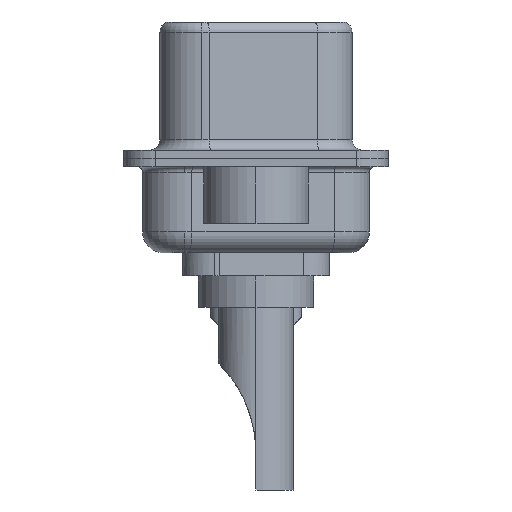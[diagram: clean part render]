
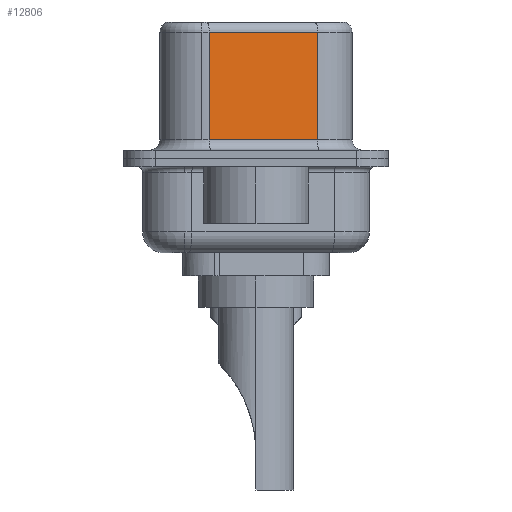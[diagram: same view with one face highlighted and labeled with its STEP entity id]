
A CAD part, left-side view. The second image highlights one B-rep face of the part: STEP entity #12806.
In plain terms, the highlighted planar face has unit normal (-0.985, -0.174, 0).
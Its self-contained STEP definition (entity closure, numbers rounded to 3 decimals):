
#2172 = CARTESIAN_POINT ( 'NONE',  ( 4.585, -2.927, 0.9 ) ) ;
#2495 = ORIENTED_EDGE ( 'NONE', *, *, #9477, .F. ) ;
#3134 = CARTESIAN_POINT ( 'NONE',  ( 3.675, 2.233, 6.02 ) ) ;
#3304 = VERTEX_POINT ( 'NONE', #3134 ) ;
#4158 = CARTESIAN_POINT ( 'NONE',  ( 4.585, -2.927, 0.9 ) ) ;
#4220 = VECTOR ( 'NONE', #18184, 1000. ) ;
#4547 = LINE ( 'NONE', #4779, #8338 ) ;
#4556 = EDGE_CURVE ( 'NONE', #10216, #3304, #4547, .T. ) ;
#4779 = CARTESIAN_POINT ( 'NONE',  ( 4.585, -2.927, 6.02 ) ) ;
#4795 = DIRECTION ( 'NONE',  ( 0.985, 0.174, 0. ) ) ;
#5337 = CARTESIAN_POINT ( 'NONE',  ( 4.585, -2.927, 6.52 ) ) ;
#7365 = DIRECTION ( 'NONE',  ( 0.174, -0.985, 0. ) ) ;
#8338 = VECTOR ( 'NONE', #15722, 1000. ) ;
#8511 = LINE ( 'NONE', #12081, #4220 ) ;
#9477 = EDGE_CURVE ( 'NONE', #10216, #18686, #19668, .T. ) ;
#10051 = ORIENTED_EDGE ( 'NONE', *, *, #4556, .T. ) ;
#10216 = VERTEX_POINT ( 'NONE', #19358 ) ;
#10341 = EDGE_CURVE ( 'NONE', #20203, #18686, #15147, .T. ) ;
#10823 = CARTESIAN_POINT ( 'NONE',  ( 3.675, 2.233, 0.9 ) ) ;
#11740 = AXIS2_PLACEMENT_3D ( 'NONE', #17172, #4795, #15715 ) ;
#12081 = CARTESIAN_POINT ( 'NONE',  ( 3.675, 2.233, 6.52 ) ) ;
#12806 = ADVANCED_FACE ( 'NONE', ( #12912 ), #14179, .F. ) ;
#12912 = FACE_OUTER_BOUND ( 'NONE', #13706, .T. ) ;
#13706 = EDGE_LOOP ( 'NONE', ( #2495, #10051, #14544, #14278 ) ) ;
#14179 = PLANE ( 'NONE',  #11740 ) ;
#14278 = ORIENTED_EDGE ( 'NONE', *, *, #10341, .T. ) ;
#14544 = ORIENTED_EDGE ( 'NONE', *, *, #16356, .T. ) ;
#15147 = LINE ( 'NONE', #4158, #19178 ) ;
#15715 = DIRECTION ( 'NONE',  ( -0.174, 0.985, 0. ) ) ;
#15722 = DIRECTION ( 'NONE',  ( -0.174, 0.985, 0. ) ) ;
#16216 = DIRECTION ( 'NONE',  ( 0., 0., -1. ) ) ;
#16356 = EDGE_CURVE ( 'NONE', #3304, #20203, #8511, .T. ) ;
#17172 = CARTESIAN_POINT ( 'NONE',  ( 4.585, -2.927, 6.52 ) ) ;
#18184 = DIRECTION ( 'NONE',  ( 0., 0., -1. ) ) ;
#18686 = VERTEX_POINT ( 'NONE', #2172 ) ;
#19178 = VECTOR ( 'NONE', #7365, 1000. ) ;
#19358 = CARTESIAN_POINT ( 'NONE',  ( 4.585, -2.927, 6.02 ) ) ;
#19668 = LINE ( 'NONE', #5337, #20158 ) ;
#20158 = VECTOR ( 'NONE', #16216, 1000. ) ;
#20203 = VERTEX_POINT ( 'NONE', #10823 ) ;
